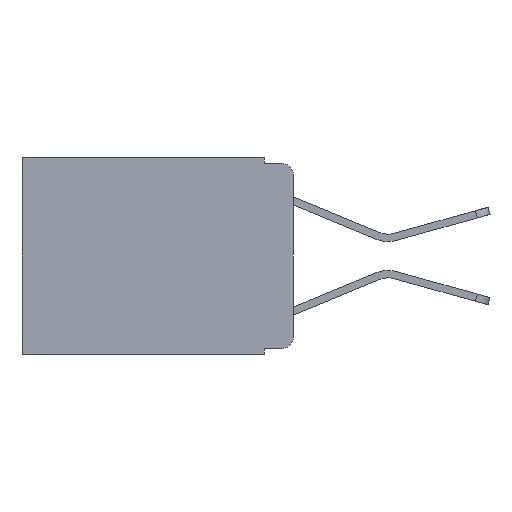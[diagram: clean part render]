
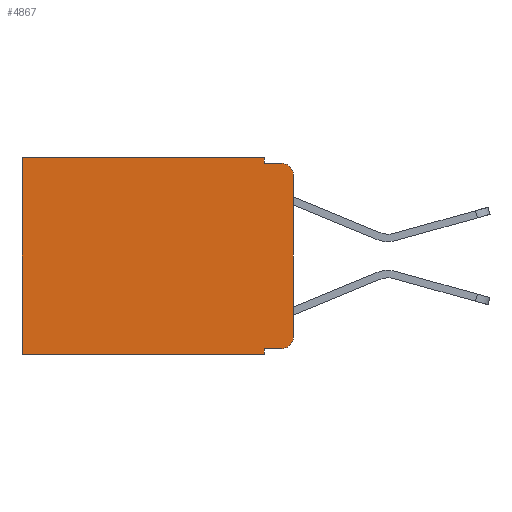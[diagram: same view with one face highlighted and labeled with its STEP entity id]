
A CAD part, left-side view. The second image highlights one B-rep face of the part: STEP entity #4867.
In plain terms, the highlighted planar face has unit normal (-1, 0, 0).
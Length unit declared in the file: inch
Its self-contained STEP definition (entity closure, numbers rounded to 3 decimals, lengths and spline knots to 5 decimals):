
#296 = CARTESIAN_POINT ( 'NONE',  ( 0.298, 0.051, -0.333 ) ) ;
#415 = CARTESIAN_POINT ( 'NONE',  ( 0.298, 0., -0.03 ) ) ;
#641 = CARTESIAN_POINT ( 'NONE',  ( 0.298, 0.473, 0. ) ) ;
#884 = EDGE_CURVE ( 'NONE', #3107, #8411, #13605, .T. ) ;
#900 = AXIS2_PLACEMENT_3D ( 'NONE', #12438, #4033, #13804 ) ;
#1031 = ORIENTED_EDGE ( 'NONE', *, *, #6225, .T. ) ;
#1073 = DIRECTION ( 'NONE',  ( 0., 1., 0. ) ) ;
#1286 = VECTOR ( 'NONE', #16177, 39.37008 ) ;
#1591 = CIRCLE ( 'NONE', #900, 0.02 ) ;
#1957 = VECTOR ( 'NONE', #1073, 39.37008 ) ;
#2008 = ORIENTED_EDGE ( 'NONE', *, *, #17605, .T. ) ;
#2138 = CIRCLE ( 'NONE', #7847, 0.02 ) ;
#2801 = CARTESIAN_POINT ( 'NONE',  ( 0.298, 0., -0.313 ) ) ;
#2832 = VERTEX_POINT ( 'NONE', #12762 ) ;
#2850 = ORIENTED_EDGE ( 'NONE', *, *, #9720, .T. ) ;
#3065 = ORIENTED_EDGE ( 'NONE', *, *, #11216, .F. ) ;
#3107 = VERTEX_POINT ( 'NONE', #641 ) ;
#3134 = PLANE ( 'NONE',  #15984 ) ;
#3181 = CARTESIAN_POINT ( 'NONE',  ( 0.298, 0.473, 0. ) ) ;
#3441 = CARTESIAN_POINT ( 'NONE',  ( 0.298, 0.02, -0.03 ) ) ;
#3604 = EDGE_CURVE ( 'NONE', #2832, #10820, #15639, .T. ) ;
#4001 = EDGE_CURVE ( 'NONE', #12943, #2832, #6622, .T. ) ;
#4033 = DIRECTION ( 'NONE',  ( -1., 0., 0. ) ) ;
#4409 = VERTEX_POINT ( 'NONE', #415 ) ;
#4822 = CARTESIAN_POINT ( 'NONE',  ( 0.298, 0.051, -0.343 ) ) ;
#4867 = ADVANCED_FACE ( 'NONE', ( #11136 ), #3134, .F. ) ;
#4975 = DIRECTION ( 'NONE',  ( 0., 0., -1. ) ) ;
#5089 = ORIENTED_EDGE ( 'NONE', *, *, #13389, .F. ) ;
#5128 = CARTESIAN_POINT ( 'NONE',  ( 0.298, 0., 0. ) ) ;
#5156 = VECTOR ( 'NONE', #5174, 39.37008 ) ;
#5174 = DIRECTION ( 'NONE',  ( 0., 1., 0. ) ) ;
#5317 = LINE ( 'NONE', #14741, #12276 ) ;
#5535 = ORIENTED_EDGE ( 'NONE', *, *, #4001, .F. ) ;
#5599 = ORIENTED_EDGE ( 'NONE', *, *, #17939, .F. ) ;
#5629 = CARTESIAN_POINT ( 'NONE',  ( 0.298, 0.051, -0.01 ) ) ;
#6137 = DIRECTION ( 'NONE',  ( 0., 0., -1. ) ) ;
#6194 = ORIENTED_EDGE ( 'NONE', *, *, #884, .T. ) ;
#6225 = EDGE_CURVE ( 'NONE', #4409, #10820, #2138, .T. ) ;
#6235 = CARTESIAN_POINT ( 'NONE',  ( 0.298, 0.02, -0.01 ) ) ;
#6309 = CARTESIAN_POINT ( 'NONE',  ( 0.298, 0.02, -0.333 ) ) ;
#6363 = DIRECTION ( 'NONE',  ( 0., 0., -1. ) ) ;
#6390 = EDGE_LOOP ( 'NONE', ( #5599, #1031, #10947, #5535, #7875, #6194, #3065, #5089, #2850, #2008 ) ) ;
#6554 = CARTESIAN_POINT ( 'NONE',  ( 0.298, 0.473, -0.343 ) ) ;
#6622 = LINE ( 'NONE', #12335, #13948 ) ;
#7847 = AXIS2_PLACEMENT_3D ( 'NONE', #3441, #13298, #4975 ) ;
#7875 = ORIENTED_EDGE ( 'NONE', *, *, #7983, .T. ) ;
#7983 = EDGE_CURVE ( 'NONE', #12943, #3107, #8920, .T. ) ;
#8411 = VERTEX_POINT ( 'NONE', #6554 ) ;
#8819 = CARTESIAN_POINT ( 'NONE',  ( 0.298, 0., 0. ) ) ;
#8920 = LINE ( 'NONE', #8819, #5156 ) ;
#9106 = LINE ( 'NONE', #16766, #12747 ) ;
#9172 = DIRECTION ( 'NONE',  ( 0., -1., 0. ) ) ;
#9508 = VERTEX_POINT ( 'NONE', #296 ) ;
#9720 = EDGE_CURVE ( 'NONE', #9508, #14390, #9106, .T. ) ;
#9963 = DIRECTION ( 'NONE',  ( 0., -1., 0. ) ) ;
#10042 = VERTEX_POINT ( 'NONE', #2801 ) ;
#10261 = CARTESIAN_POINT ( 'NONE',  ( 0.298, 0., 0. ) ) ;
#10820 = VERTEX_POINT ( 'NONE', #6235 ) ;
#10947 = ORIENTED_EDGE ( 'NONE', *, *, #3604, .F. ) ;
#11136 = FACE_OUTER_BOUND ( 'NONE', #6390, .T. ) ;
#11187 = CARTESIAN_POINT ( 'NONE',  ( 0.298, 0., -0.343 ) ) ;
#11216 = EDGE_CURVE ( 'NONE', #11364, #8411, #12461, .T. ) ;
#11364 = VERTEX_POINT ( 'NONE', #4822 ) ;
#12276 = VECTOR ( 'NONE', #16128, 39.37008 ) ;
#12335 = CARTESIAN_POINT ( 'NONE',  ( 0.298, 0.051, 0. ) ) ;
#12438 = CARTESIAN_POINT ( 'NONE',  ( 0.298, 0.02, -0.313 ) ) ;
#12461 = LINE ( 'NONE', #11187, #1957 ) ;
#12726 = LINE ( 'NONE', #5128, #1286 ) ;
#12747 = VECTOR ( 'NONE', #9172, 39.37008 ) ;
#12761 = VECTOR ( 'NONE', #16452, 39.37008 ) ;
#12762 = CARTESIAN_POINT ( 'NONE',  ( 0.298, 0.051, -0.01 ) ) ;
#12943 = VERTEX_POINT ( 'NONE', #17809 ) ;
#13298 = DIRECTION ( 'NONE',  ( -1., 0., 0. ) ) ;
#13389 = EDGE_CURVE ( 'NONE', #9508, #11364, #5317, .T. ) ;
#13605 = LINE ( 'NONE', #3181, #12761 ) ;
#13804 = DIRECTION ( 'NONE',  ( 0., 0., -1. ) ) ;
#13948 = VECTOR ( 'NONE', #6363, 39.37008 ) ;
#14376 = DIRECTION ( 'NONE',  ( 1., 0., 0. ) ) ;
#14390 = VERTEX_POINT ( 'NONE', #6309 ) ;
#14741 = CARTESIAN_POINT ( 'NONE',  ( 0.298, 0.051, 0. ) ) ;
#15204 = VECTOR ( 'NONE', #9963, 39.37008 ) ;
#15639 = LINE ( 'NONE', #5629, #15204 ) ;
#15984 = AXIS2_PLACEMENT_3D ( 'NONE', #10261, #14376, #6137 ) ;
#16128 = DIRECTION ( 'NONE',  ( 0., 0., -1. ) ) ;
#16177 = DIRECTION ( 'NONE',  ( 0., 0., -1. ) ) ;
#16452 = DIRECTION ( 'NONE',  ( 0., 0., -1. ) ) ;
#16766 = CARTESIAN_POINT ( 'NONE',  ( 0.298, 0.051, -0.333 ) ) ;
#17605 = EDGE_CURVE ( 'NONE', #14390, #10042, #1591, .T. ) ;
#17809 = CARTESIAN_POINT ( 'NONE',  ( 0.298, 0.051, 0. ) ) ;
#17939 = EDGE_CURVE ( 'NONE', #4409, #10042, #12726, .T. ) ;
